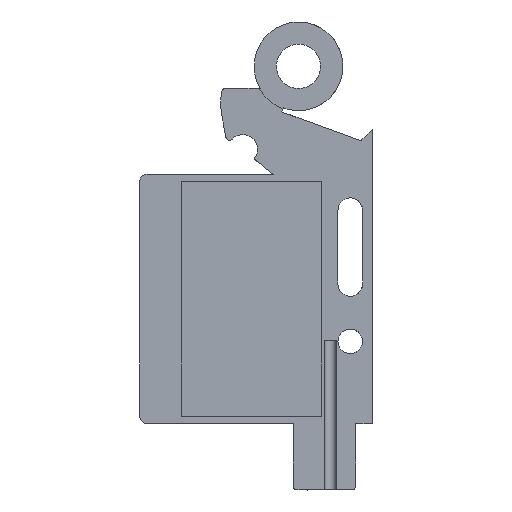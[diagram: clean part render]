
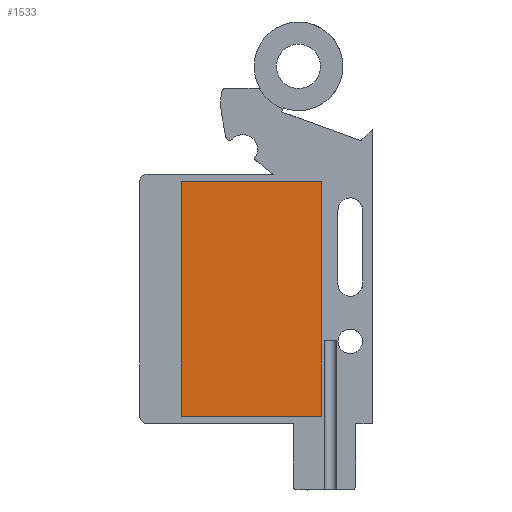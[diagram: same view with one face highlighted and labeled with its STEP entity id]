
A CAD part, left-side view. The second image highlights one B-rep face of the part: STEP entity #1533.
In plain terms, the highlighted planar face has unit normal (-1, 0, 0).
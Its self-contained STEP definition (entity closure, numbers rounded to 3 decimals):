
#128 = EDGE_CURVE ( 'NONE', #3977, #1671, #2595, .T. ) ;
#156 = DIRECTION ( 'NONE',  ( 0., 0., -1. ) ) ;
#159 = CARTESIAN_POINT ( 'NONE',  ( 11.525, 1., 24.875 ) ) ;
#214 = EDGE_CURVE ( 'NONE', #1449, #3977, #3352, .T. ) ;
#325 = EDGE_CURVE ( 'NONE', #1805, #1449, #1225, .T. ) ;
#404 = EDGE_CURVE ( 'NONE', #1805, #1671, #2888, .T. ) ;
#661 = VECTOR ( 'NONE', #156, 1000. ) ;
#1124 = FACE_OUTER_BOUND ( 'NONE', #2567, .T. ) ;
#1220 = DIRECTION ( 'NONE',  ( 0., -1., 0. ) ) ;
#1225 = LINE ( 'NONE', #3143, #3123 ) ;
#1449 = VERTEX_POINT ( 'NONE', #4936 ) ;
#1533 = ADVANCED_FACE ( 'NONE', ( #1124 ), #1619, .F. ) ;
#1619 = PLANE ( 'NONE',  #2994 ) ;
#1671 = VERTEX_POINT ( 'NONE', #2613 ) ;
#1694 = CARTESIAN_POINT ( 'NONE',  ( 11.525, 10.525, 40.75 ) ) ;
#1792 = CARTESIAN_POINT ( 'NONE',  ( 11.525, 20.05, 9. ) ) ;
#1805 = VERTEX_POINT ( 'NONE', #1792 ) ;
#1989 = ORIENTED_EDGE ( 'NONE', *, *, #325, .F. ) ;
#2116 = ORIENTED_EDGE ( 'NONE', *, *, #404, .T. ) ;
#2369 = VECTOR ( 'NONE', #1220, 1000. ) ;
#2385 = DIRECTION ( 'NONE',  ( 0., 0., 1. ) ) ;
#2567 = EDGE_LOOP ( 'NONE', ( #3261, #4657, #1989, #2116 ) ) ;
#2595 = LINE ( 'NONE', #159, #661 ) ;
#2613 = CARTESIAN_POINT ( 'NONE',  ( 11.525, 1., 9. ) ) ;
#2888 = LINE ( 'NONE', #3797, #4744 ) ;
#2994 = AXIS2_PLACEMENT_3D ( 'NONE', #4239, #4610, #2385 ) ;
#3081 = DIRECTION ( 'NONE',  ( 0., -1., 0. ) ) ;
#3123 = VECTOR ( 'NONE', #3500, 1000. ) ;
#3143 = CARTESIAN_POINT ( 'NONE',  ( 11.525, 20.05, 24.875 ) ) ;
#3261 = ORIENTED_EDGE ( 'NONE', *, *, #128, .F. ) ;
#3352 = LINE ( 'NONE', #1694, #2369 ) ;
#3500 = DIRECTION ( 'NONE',  ( 0., 0., 1. ) ) ;
#3797 = CARTESIAN_POINT ( 'NONE',  ( 11.525, 10.525, 9. ) ) ;
#3977 = VERTEX_POINT ( 'NONE', #4757 ) ;
#4239 = CARTESIAN_POINT ( 'NONE',  ( 11.525, 1., 9. ) ) ;
#4610 = DIRECTION ( 'NONE',  ( 1., 0., 0. ) ) ;
#4657 = ORIENTED_EDGE ( 'NONE', *, *, #214, .F. ) ;
#4744 = VECTOR ( 'NONE', #3081, 1000. ) ;
#4757 = CARTESIAN_POINT ( 'NONE',  ( 11.525, 1., 40.75 ) ) ;
#4936 = CARTESIAN_POINT ( 'NONE',  ( 11.525, 20.05, 40.75 ) ) ;
